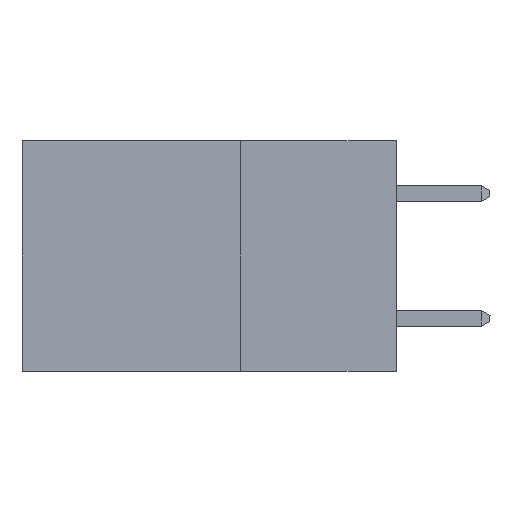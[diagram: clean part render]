
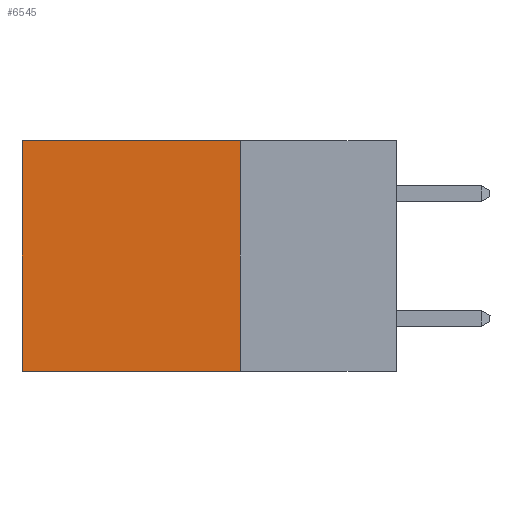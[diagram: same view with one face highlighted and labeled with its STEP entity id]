
A CAD part, left-side view. The second image highlights one B-rep face of the part: STEP entity #6545.
In plain terms, the highlighted planar face has unit normal (-1, 0, 0).
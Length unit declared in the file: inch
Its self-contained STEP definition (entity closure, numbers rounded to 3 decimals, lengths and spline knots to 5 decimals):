
#594 = EDGE_LOOP ( 'NONE', ( #5526, #18120, #19099, #8776 ) ) ;
#830 = FACE_OUTER_BOUND ( 'NONE', #594, .T. ) ;
#1189 = CARTESIAN_POINT ( 'NONE',  ( 0.298, 0.25, -0.37 ) ) ;
#1768 = LINE ( 'NONE', #25332, #12175 ) ;
#3861 = CARTESIAN_POINT ( 'NONE',  ( 0.298, 0.25, 0. ) ) ;
#4381 = VERTEX_POINT ( 'NONE', #15712 ) ;
#5526 = ORIENTED_EDGE ( 'NONE', *, *, #20766, .T. ) ;
#5990 = EDGE_CURVE ( 'NONE', #8190, #10530, #1768, .T. ) ;
#6545 = ADVANCED_FACE ( 'NONE', ( #830 ), #15524, .F. ) ;
#6918 = VECTOR ( 'NONE', #8498, 39.37008 ) ;
#7314 = LINE ( 'NONE', #15613, #9442 ) ;
#7712 = EDGE_CURVE ( 'NONE', #16443, #4381, #12434, .T. ) ;
#8190 = VERTEX_POINT ( 'NONE', #17500 ) ;
#8498 = DIRECTION ( 'NONE',  ( 0., 0., -1. ) ) ;
#8776 = ORIENTED_EDGE ( 'NONE', *, *, #5990, .T. ) ;
#9204 = AXIS2_PLACEMENT_3D ( 'NONE', #3861, #19578, #19502 ) ;
#9442 = VECTOR ( 'NONE', #11492, 39.37008 ) ;
#10530 = VERTEX_POINT ( 'NONE', #17278 ) ;
#11492 = DIRECTION ( 'NONE',  ( 0., 0., -1. ) ) ;
#11566 = DIRECTION ( 'NONE',  ( 0., 1., 0. ) ) ;
#12175 = VECTOR ( 'NONE', #23433, 39.37008 ) ;
#12434 = LINE ( 'NONE', #21596, #21724 ) ;
#15524 = PLANE ( 'NONE',  #9204 ) ;
#15613 = CARTESIAN_POINT ( 'NONE',  ( 0.298, 0.25, 0. ) ) ;
#15712 = CARTESIAN_POINT ( 'NONE',  ( 0.298, 0.6, -0.37 ) ) ;
#16443 = VERTEX_POINT ( 'NONE', #1189 ) ;
#17278 = CARTESIAN_POINT ( 'NONE',  ( 0.298, 0.6, 0. ) ) ;
#17500 = CARTESIAN_POINT ( 'NONE',  ( 0.298, 0.25, 0. ) ) ;
#18120 = ORIENTED_EDGE ( 'NONE', *, *, #7712, .F. ) ;
#19099 = ORIENTED_EDGE ( 'NONE', *, *, #19376, .F. ) ;
#19376 = EDGE_CURVE ( 'NONE', #8190, #16443, #7314, .T. ) ;
#19502 = DIRECTION ( 'NONE',  ( 0., 0., -1. ) ) ;
#19578 = DIRECTION ( 'NONE',  ( 1., 0., 0. ) ) ;
#20414 = CARTESIAN_POINT ( 'NONE',  ( 0.298, 0.6, 0. ) ) ;
#20766 = EDGE_CURVE ( 'NONE', #10530, #4381, #23283, .T. ) ;
#21596 = CARTESIAN_POINT ( 'NONE',  ( 0.298, 0.25, -0.37 ) ) ;
#21724 = VECTOR ( 'NONE', #11566, 39.37008 ) ;
#23283 = LINE ( 'NONE', #20414, #6918 ) ;
#23433 = DIRECTION ( 'NONE',  ( 0., 1., 0. ) ) ;
#25332 = CARTESIAN_POINT ( 'NONE',  ( 0.298, 0.25, 0. ) ) ;
